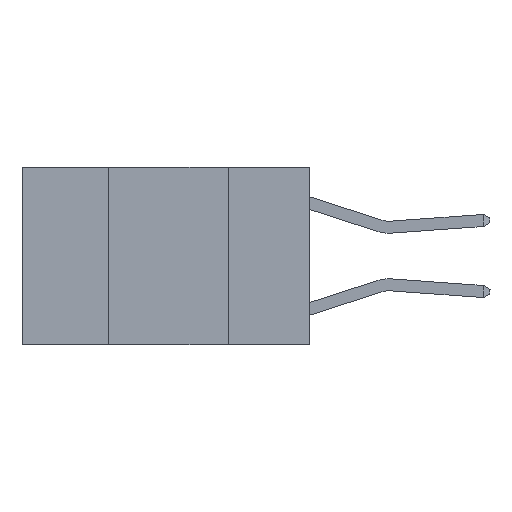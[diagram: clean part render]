
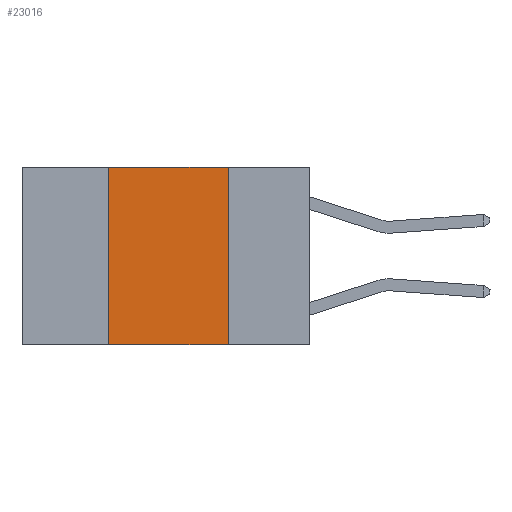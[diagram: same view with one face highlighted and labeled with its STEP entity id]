
A CAD part, left-side view. The second image highlights one B-rep face of the part: STEP entity #23016.
In plain terms, the highlighted planar face has unit normal (-1, 0, 0).
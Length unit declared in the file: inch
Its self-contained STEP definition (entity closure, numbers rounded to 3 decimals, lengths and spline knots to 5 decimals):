
#238 = CARTESIAN_POINT ( 'NONE',  ( 0., 0.6, -0.37 ) ) ;
#1559 = EDGE_CURVE ( 'NONE', #14849, #1569, #16085, .T. ) ;
#1569 = VERTEX_POINT ( 'NONE', #17841 ) ;
#1739 = ORIENTED_EDGE ( 'NONE', *, *, #18790, .F. ) ;
#3260 = LINE ( 'NONE', #13456, #19015 ) ;
#3587 = EDGE_CURVE ( 'NONE', #1569, #23109, #7731, .T. ) ;
#5580 = DIRECTION ( 'NONE',  ( 0., 0., -1. ) ) ;
#6511 = PLANE ( 'NONE',  #17386 ) ;
#6645 = DIRECTION ( 'NONE',  ( 0., 0., -1. ) ) ;
#7731 = LINE ( 'NONE', #10000, #9016 ) ;
#7894 = VECTOR ( 'NONE', #18763, 39.37008 ) ;
#9016 = VECTOR ( 'NONE', #5580, 39.37008 ) ;
#9068 = CARTESIAN_POINT ( 'NONE',  ( 0., 0.42, -0.37 ) ) ;
#10000 = CARTESIAN_POINT ( 'NONE',  ( 0., 0.17, 0. ) ) ;
#10049 = DIRECTION ( 'NONE',  ( 0., -1., 0. ) ) ;
#11105 = LINE ( 'NONE', #238, #7894 ) ;
#13456 = CARTESIAN_POINT ( 'NONE',  ( 0., 0.42, 0. ) ) ;
#13805 = CARTESIAN_POINT ( 'NONE',  ( 0., 0.6, 0. ) ) ;
#14106 = ORIENTED_EDGE ( 'NONE', *, *, #1559, .F. ) ;
#14680 = DIRECTION ( 'NONE',  ( 1., 0., 0. ) ) ;
#14849 = VERTEX_POINT ( 'NONE', #18362 ) ;
#16085 = LINE ( 'NONE', #13805, #25705 ) ;
#17386 = AXIS2_PLACEMENT_3D ( 'NONE', #25030, #14680, #6645 ) ;
#17841 = CARTESIAN_POINT ( 'NONE',  ( 0., 0.17, 0. ) ) ;
#18362 = CARTESIAN_POINT ( 'NONE',  ( 0., 0.42, 0. ) ) ;
#18375 = VERTEX_POINT ( 'NONE', #9068 ) ;
#18763 = DIRECTION ( 'NONE',  ( 0., -1., 0. ) ) ;
#18790 = EDGE_CURVE ( 'NONE', #18375, #14849, #3260, .T. ) ;
#19015 = VECTOR ( 'NONE', #25417, 39.37008 ) ;
#19481 = EDGE_CURVE ( 'NONE', #18375, #23109, #11105, .T. ) ;
#19776 = ORIENTED_EDGE ( 'NONE', *, *, #19481, .T. ) ;
#21115 = FACE_OUTER_BOUND ( 'NONE', #24228, .T. ) ;
#23016 = ADVANCED_FACE ( 'NONE', ( #21115 ), #6511, .F. ) ;
#23109 = VERTEX_POINT ( 'NONE', #23800 ) ;
#23688 = ORIENTED_EDGE ( 'NONE', *, *, #3587, .F. ) ;
#23800 = CARTESIAN_POINT ( 'NONE',  ( 0., 0.17, -0.37 ) ) ;
#24228 = EDGE_LOOP ( 'NONE', ( #23688, #14106, #1739, #19776 ) ) ;
#25030 = CARTESIAN_POINT ( 'NONE',  ( 0., 0.6, 0. ) ) ;
#25417 = DIRECTION ( 'NONE',  ( 0., 0., 1. ) ) ;
#25705 = VECTOR ( 'NONE', #10049, 39.37008 ) ;
